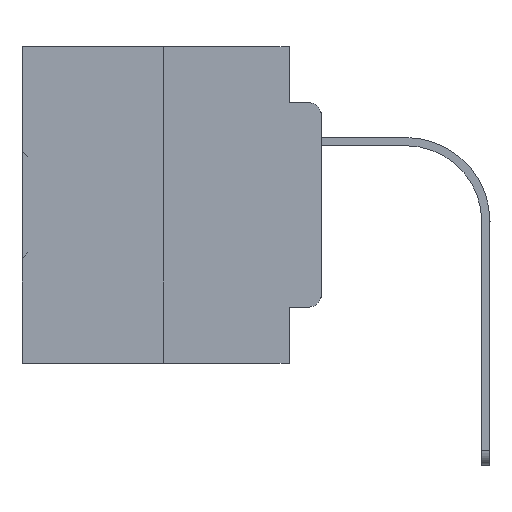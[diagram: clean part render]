
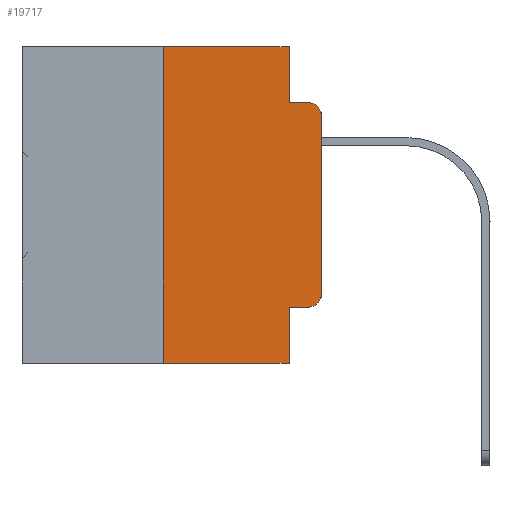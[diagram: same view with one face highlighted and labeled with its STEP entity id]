
A CAD part, left-side view. The second image highlights one B-rep face of the part: STEP entity #19717.
In plain terms, the highlighted planar face has unit normal (-1, 0, 0).
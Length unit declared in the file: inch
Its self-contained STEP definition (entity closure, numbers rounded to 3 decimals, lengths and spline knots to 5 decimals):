
#202 = ORIENTED_EDGE ( 'NONE', *, *, #3586, .T. ) ;
#1908 = EDGE_CURVE ( 'NONE', #18379, #30644, #23691, .T. ) ;
#2090 = CARTESIAN_POINT ( 'NONE',  ( 0., 0.051, -0.4115 ) ) ;
#2137 = CARTESIAN_POINT ( 'NONE',  ( 0., 0., 0. ) ) ;
#2357 = DIRECTION ( 'NONE',  ( -1., 0., 0. ) ) ;
#2432 = FACE_OUTER_BOUND ( 'NONE', #26505, .T. ) ;
#2453 = VERTEX_POINT ( 'NONE', #2868 ) ;
#2500 = CARTESIAN_POINT ( 'NONE',  ( 0., 0.25, 0. ) ) ;
#2657 = CARTESIAN_POINT ( 'NONE',  ( 0., 0., -0.1085 ) ) ;
#2743 = CARTESIAN_POINT ( 'NONE',  ( 0., 0.051, -0.5 ) ) ;
#2786 = PLANE ( 'NONE',  #15576 ) ;
#2868 = CARTESIAN_POINT ( 'NONE',  ( 0., 0.051, 0. ) ) ;
#2910 = DIRECTION ( 'NONE',  ( 0., -1., 0. ) ) ;
#3210 = CARTESIAN_POINT ( 'NONE',  ( 0., 0.473, -0.5 ) ) ;
#3586 = EDGE_CURVE ( 'NONE', #19356, #7011, #6967, .T. ) ;
#4030 = VERTEX_POINT ( 'NONE', #2500 ) ;
#4966 = VECTOR ( 'NONE', #15802, 39.37008 ) ;
#5374 = VECTOR ( 'NONE', #26960, 39.37008 ) ;
#5396 = ORIENTED_EDGE ( 'NONE', *, *, #1908, .F. ) ;
#5442 = DIRECTION ( 'NONE',  ( 0., 0., -1. ) ) ;
#5445 = DIRECTION ( 'NONE',  ( -1., 0., 0. ) ) ;
#5587 = CARTESIAN_POINT ( 'NONE',  ( 0., 0.051, -0.0885 ) ) ;
#6135 = ORIENTED_EDGE ( 'NONE', *, *, #17681, .T. ) ;
#6427 = CARTESIAN_POINT ( 'NONE',  ( 0., 0., -0.3915 ) ) ;
#6905 = ORIENTED_EDGE ( 'NONE', *, *, #16812, .T. ) ;
#6967 = CIRCLE ( 'NONE', #26769, 0.02 ) ;
#7011 = VERTEX_POINT ( 'NONE', #12632 ) ;
#8014 = VECTOR ( 'NONE', #29765, 39.37008 ) ;
#8254 = LINE ( 'NONE', #5587, #11964 ) ;
#9962 = ORIENTED_EDGE ( 'NONE', *, *, #30214, .T. ) ;
#10456 = VECTOR ( 'NONE', #29349, 39.37008 ) ;
#10583 = CARTESIAN_POINT ( 'NONE',  ( 0., 0.473, 0. ) ) ;
#10672 = VERTEX_POINT ( 'NONE', #20633 ) ;
#11964 = VECTOR ( 'NONE', #2910, 39.37008 ) ;
#12632 = CARTESIAN_POINT ( 'NONE',  ( 0., 0.02, -0.0885 ) ) ;
#13167 = CARTESIAN_POINT ( 'NONE',  ( 0., 0.051, 0. ) ) ;
#13840 = DIRECTION ( 'NONE',  ( 0., -1., 0. ) ) ;
#15576 = AXIS2_PLACEMENT_3D ( 'NONE', #10583, #29727, #5442 ) ;
#15578 = VERTEX_POINT ( 'NONE', #6427 ) ;
#15802 = DIRECTION ( 'NONE',  ( 0., -1., 0. ) ) ;
#15814 = EDGE_CURVE ( 'NONE', #18379, #23199, #32290, .T. ) ;
#15824 = CARTESIAN_POINT ( 'NONE',  ( 0., 0.02, -0.1085 ) ) ;
#15825 = LINE ( 'NONE', #13167, #32435 ) ;
#16050 = EDGE_CURVE ( 'NONE', #10672, #4030, #28549, .T. ) ;
#16253 = DIRECTION ( 'NONE',  ( 0., 0., -1. ) ) ;
#16812 = EDGE_CURVE ( 'NONE', #23199, #15578, #22871, .T. ) ;
#16853 = LINE ( 'NONE', #34953, #20170 ) ;
#17681 = EDGE_CURVE ( 'NONE', #10672, #30644, #21821, .T. ) ;
#18230 = LINE ( 'NONE', #2137, #8014 ) ;
#18379 = VERTEX_POINT ( 'NONE', #2090 ) ;
#18961 = ORIENTED_EDGE ( 'NONE', *, *, #24564, .F. ) ;
#18965 = EDGE_CURVE ( 'NONE', #4030, #2453, #16853, .T. ) ;
#19356 = VERTEX_POINT ( 'NONE', #2657 ) ;
#19717 = ADVANCED_FACE ( 'NONE', ( #2432 ), #2786, .F. ) ;
#20037 = CARTESIAN_POINT ( 'NONE',  ( 0., 0.25, 0. ) ) ;
#20170 = VECTOR ( 'NONE', #13840, 39.37008 ) ;
#20633 = CARTESIAN_POINT ( 'NONE',  ( 0., 0.25, -0.5 ) ) ;
#21821 = LINE ( 'NONE', #3210, #5374 ) ;
#22723 = EDGE_CURVE ( 'NONE', #31722, #7011, #8254, .T. ) ;
#22871 = CIRCLE ( 'NONE', #31380, 0.02 ) ;
#23199 = VERTEX_POINT ( 'NONE', #29465 ) ;
#23691 = LINE ( 'NONE', #32023, #10456 ) ;
#24564 = EDGE_CURVE ( 'NONE', #2453, #31722, #15825, .T. ) ;
#24908 = CARTESIAN_POINT ( 'NONE',  ( 0., 0.02, -0.3915 ) ) ;
#25942 = VECTOR ( 'NONE', #28887, 39.37008 ) ;
#26505 = EDGE_LOOP ( 'NONE', ( #9962, #202, #32843, #18961, #28075, #29234, #6135, #5396, #29858, #6905 ) ) ;
#26769 = AXIS2_PLACEMENT_3D ( 'NONE', #15824, #2357, #34808 ) ;
#26960 = DIRECTION ( 'NONE',  ( 0., -1., 0. ) ) ;
#26969 = CARTESIAN_POINT ( 'NONE',  ( 0., 0.051, -0.4115 ) ) ;
#28075 = ORIENTED_EDGE ( 'NONE', *, *, #18965, .F. ) ;
#28549 = LINE ( 'NONE', #20037, #25942 ) ;
#28887 = DIRECTION ( 'NONE',  ( 0., 0., 1. ) ) ;
#29234 = ORIENTED_EDGE ( 'NONE', *, *, #16050, .F. ) ;
#29349 = DIRECTION ( 'NONE',  ( 0., 0., -1. ) ) ;
#29465 = CARTESIAN_POINT ( 'NONE',  ( 0., 0.02, -0.4115 ) ) ;
#29727 = DIRECTION ( 'NONE',  ( 1., 0., 0. ) ) ;
#29765 = DIRECTION ( 'NONE',  ( 0., 0., 1. ) ) ;
#29858 = ORIENTED_EDGE ( 'NONE', *, *, #15814, .T. ) ;
#30214 = EDGE_CURVE ( 'NONE', #15578, #19356, #18230, .T. ) ;
#30644 = VERTEX_POINT ( 'NONE', #2743 ) ;
#31380 = AXIS2_PLACEMENT_3D ( 'NONE', #24908, #5445, #16253 ) ;
#31722 = VERTEX_POINT ( 'NONE', #34191 ) ;
#32023 = CARTESIAN_POINT ( 'NONE',  ( 0., 0.051, 0. ) ) ;
#32290 = LINE ( 'NONE', #26969, #4966 ) ;
#32435 = VECTOR ( 'NONE', #34809, 39.37008 ) ;
#32843 = ORIENTED_EDGE ( 'NONE', *, *, #22723, .F. ) ;
#34191 = CARTESIAN_POINT ( 'NONE',  ( 0., 0.051, -0.0885 ) ) ;
#34808 = DIRECTION ( 'NONE',  ( 0., 0., -1. ) ) ;
#34809 = DIRECTION ( 'NONE',  ( 0., 0., -1. ) ) ;
#34953 = CARTESIAN_POINT ( 'NONE',  ( 0., 0.473, 0. ) ) ;
